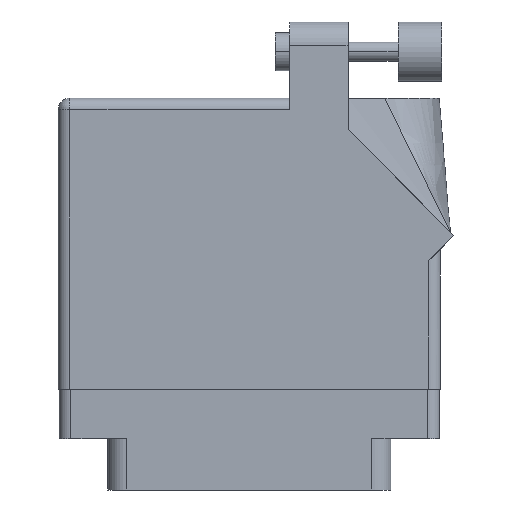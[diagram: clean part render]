
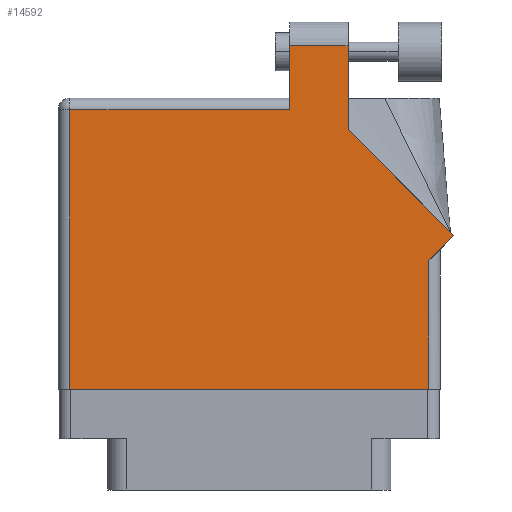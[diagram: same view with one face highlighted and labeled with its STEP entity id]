
A CAD part, front view. The second image highlights one B-rep face of the part: STEP entity #14592.
In plain terms, the highlighted face is planar.
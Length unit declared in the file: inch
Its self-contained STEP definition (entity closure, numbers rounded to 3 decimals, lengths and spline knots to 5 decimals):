
#700 = VERTEX_POINT ( 'NONE', #27052 ) ;
#1010 = LINE ( 'NONE', #33199, #28848 ) ;
#1729 = VECTOR ( 'NONE', #28286, 39.37008 ) ;
#1884 = ORIENTED_EDGE ( 'NONE', *, *, #20984, .T. ) ;
#2118 = DIRECTION ( 'NONE',  ( 0., 1., 0. ) ) ;
#2710 = EDGE_CURVE ( 'NONE', #34888, #14499, #23245, .T. ) ;
#2849 = CARTESIAN_POINT ( 'NONE',  ( 0.062, 0., 0. ) ) ;
#2995 = VERTEX_POINT ( 'NONE', #11596 ) ;
#3257 = LINE ( 'NONE', #9904, #11689 ) ;
#3797 = ORIENTED_EDGE ( 'NONE', *, *, #15639, .T. ) ;
#4353 = EDGE_CURVE ( 'NONE', #21264, #2995, #9582, .T. ) ;
#4497 = EDGE_CURVE ( 'NONE', #2995, #700, #4504, .T. ) ;
#4504 = LINE ( 'NONE', #4525, #24367 ) ;
#4525 = CARTESIAN_POINT ( 'NONE',  ( 0., 1.468, 0. ) ) ;
#6000 = DIRECTION ( 'NONE',  ( 0., -1., 0. ) ) ;
#6188 = VECTOR ( 'NONE', #17681, 39.37008 ) ;
#6841 = EDGE_CURVE ( 'NONE', #14499, #23666, #1010, .T. ) ;
#7946 = AXIS2_PLACEMENT_3D ( 'NONE', #31815, #21109, #10693 ) ;
#7955 = VECTOR ( 'NONE', #6000, 39.37008 ) ;
#8836 = CARTESIAN_POINT ( 'NONE',  ( 1.948, 0.675, 0. ) ) ;
#8853 = VERTEX_POINT ( 'NONE', #16364 ) ;
#9582 = LINE ( 'NONE', #26039, #6188 ) ;
#9904 = CARTESIAN_POINT ( 'NONE',  ( 1.217, 1.805, 0. ) ) ;
#10693 = DIRECTION ( 'NONE',  ( -1., 0., 0. ) ) ;
#11357 = ORIENTED_EDGE ( 'NONE', *, *, #17097, .T. ) ;
#11596 = CARTESIAN_POINT ( 'NONE',  ( 1.217, 1.468, 0. ) ) ;
#11689 = VECTOR ( 'NONE', #15240, 39.37008 ) ;
#12301 = ORIENTED_EDGE ( 'NONE', *, *, #4353, .T. ) ;
#12346 = VERTEX_POINT ( 'NONE', #15409 ) ;
#13100 = DIRECTION ( 'NONE',  ( 0.707, 0.707, 0. ) ) ;
#14499 = VERTEX_POINT ( 'NONE', #20874 ) ;
#14592 = ADVANCED_FACE ( 'NONE', ( #25719 ), #26889, .F. ) ;
#14601 = DIRECTION ( 'NONE',  ( -0.707, 0.707, 0. ) ) ;
#14677 = DIRECTION ( 'NONE',  ( 0., 1., 0. ) ) ;
#15240 = DIRECTION ( 'NONE',  ( -1., 0., 0. ) ) ;
#15409 = CARTESIAN_POINT ( 'NONE',  ( 1.524, 1.805, 0. ) ) ;
#15463 = CARTESIAN_POINT ( 'NONE',  ( 2.01, 0.737, 0. ) ) ;
#15639 = EDGE_CURVE ( 'NONE', #27009, #12346, #20568, .T. ) ;
#16364 = CARTESIAN_POINT ( 'NONE',  ( 2.08071, 0.80771, 0. ) ) ;
#16607 = EDGE_LOOP ( 'NONE', ( #3797, #16665, #12301, #17162, #1884, #19984, #29721, #20174, #11357 ) ) ;
#16665 = ORIENTED_EDGE ( 'NONE', *, *, #33862, .T. ) ;
#16894 = CARTESIAN_POINT ( 'NONE',  ( 0.062, 0., 0. ) ) ;
#17097 = EDGE_CURVE ( 'NONE', #8853, #27009, #22976, .T. ) ;
#17162 = ORIENTED_EDGE ( 'NONE', *, *, #4497, .T. ) ;
#17681 = DIRECTION ( 'NONE',  ( 0., -1., 0. ) ) ;
#19984 = ORIENTED_EDGE ( 'NONE', *, *, #2710, .T. ) ;
#20174 = ORIENTED_EDGE ( 'NONE', *, *, #32618, .T. ) ;
#20432 = CARTESIAN_POINT ( 'NONE',  ( 1.217, 1.805, 0. ) ) ;
#20568 = LINE ( 'NONE', #20883, #26491 ) ;
#20874 = CARTESIAN_POINT ( 'NONE',  ( 1.948, 0., 0. ) ) ;
#20883 = CARTESIAN_POINT ( 'NONE',  ( 1.524, 1.36442, 0. ) ) ;
#20984 = EDGE_CURVE ( 'NONE', #700, #34888, #23588, .T. ) ;
#21109 = DIRECTION ( 'NONE',  ( 0., 0., -1. ) ) ;
#21264 = VERTEX_POINT ( 'NONE', #20432 ) ;
#21733 = VECTOR ( 'NONE', #14601, 39.37008 ) ;
#22976 = LINE ( 'NONE', #28085, #21733 ) ;
#23245 = LINE ( 'NONE', #30736, #1729 ) ;
#23588 = LINE ( 'NONE', #16894, #7955 ) ;
#23666 = VERTEX_POINT ( 'NONE', #8836 ) ;
#24367 = VECTOR ( 'NONE', #28859, 39.37008 ) ;
#25719 = FACE_OUTER_BOUND ( 'NONE', #16607, .T. ) ;
#26039 = CARTESIAN_POINT ( 'NONE',  ( 1.217, 1.53, 0. ) ) ;
#26380 = CARTESIAN_POINT ( 'NONE',  ( 1.524, 1.36442, 0. ) ) ;
#26491 = VECTOR ( 'NONE', #2118, 39.37008 ) ;
#26889 = PLANE ( 'NONE',  #7946 ) ;
#27009 = VERTEX_POINT ( 'NONE', #26380 ) ;
#27052 = CARTESIAN_POINT ( 'NONE',  ( 0.062, 1.468, 0. ) ) ;
#28085 = CARTESIAN_POINT ( 'NONE',  ( 2.08071, 0.80771, 0. ) ) ;
#28286 = DIRECTION ( 'NONE',  ( 1., 0., 0. ) ) ;
#28848 = VECTOR ( 'NONE', #14677, 39.37008 ) ;
#28859 = DIRECTION ( 'NONE',  ( -1., 0., 0. ) ) ;
#29721 = ORIENTED_EDGE ( 'NONE', *, *, #6841, .T. ) ;
#30418 = LINE ( 'NONE', #15463, #31664 ) ;
#30736 = CARTESIAN_POINT ( 'NONE',  ( 0., 0., 0. ) ) ;
#31664 = VECTOR ( 'NONE', #13100, 39.37008 ) ;
#31815 = CARTESIAN_POINT ( 'NONE',  ( 0., 1.53, 0. ) ) ;
#32618 = EDGE_CURVE ( 'NONE', #23666, #8853, #30418, .T. ) ;
#33199 = CARTESIAN_POINT ( 'NONE',  ( 1.948, 0.737, 0. ) ) ;
#33862 = EDGE_CURVE ( 'NONE', #12346, #21264, #3257, .T. ) ;
#34888 = VERTEX_POINT ( 'NONE', #2849 ) ;
